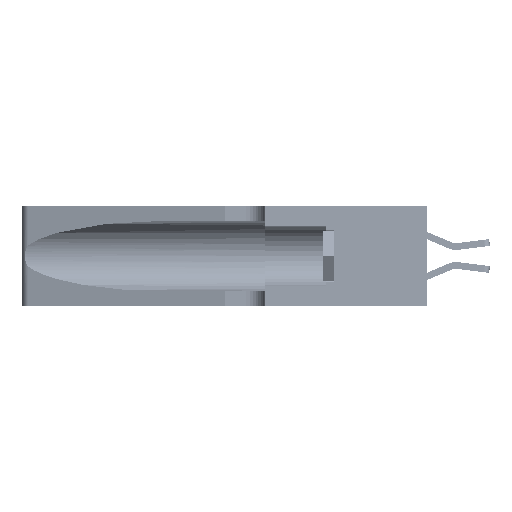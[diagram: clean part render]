
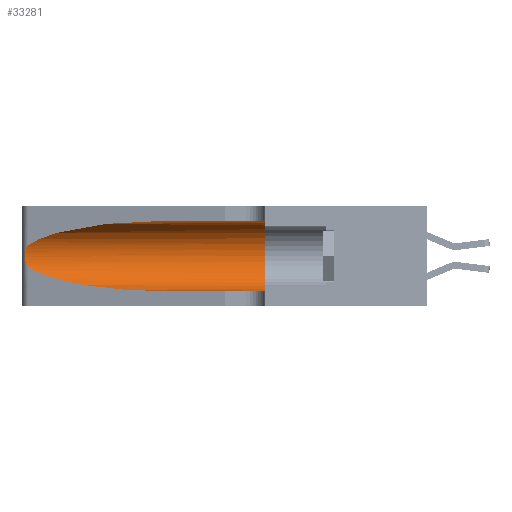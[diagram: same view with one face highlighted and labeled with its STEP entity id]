
A CAD part, left-side view. The second image highlights one B-rep face of the part: STEP entity #33281.
In plain terms, the highlighted cylindrical face has radius 3.308 mm (diameter 6.617 mm), a partial arc.
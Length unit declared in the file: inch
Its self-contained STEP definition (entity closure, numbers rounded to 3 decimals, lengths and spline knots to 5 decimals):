
#544 = VERTEX_POINT ( 'NONE', #6741 ) ;
#1522 = CARTESIAN_POINT ( 'NONE',  ( 0.25787, 1.23484, 0.2124 ) ) ;
#1813 = VERTEX_POINT ( 'NONE', #9544 ) ;
#2002 = CARTESIAN_POINT ( 'NONE',  ( 0.25487, 1.22718, 0.14631 ) ) ;
#2209 = ORIENTED_EDGE ( 'NONE', *, *, #15347, .T. ) ;
#2214 = VERTEX_POINT ( 'NONE', #2002 ) ;
#3667 = ORIENTED_EDGE ( 'NONE', *, *, #12165, .F. ) ;
#4378 = CARTESIAN_POINT ( 'NONE',  ( 0.18966, 0.96281, 0.05475 ) ) ;
#4604 = CARTESIAN_POINT ( 'NONE',  ( 0.26018, 1.23835, 0.19895 ) ) ;
#4618 = CARTESIAN_POINT ( 'NONE',  ( 0.2373, 1.15595, 0.28018 ) ) ;
#5197 = LINE ( 'NONE', #16268, #27668 ) ;
#6741 = CARTESIAN_POINT ( 'NONE',  ( 0.1305, 0.35, 0.05475 ) ) ;
#6947 = ORIENTED_EDGE ( 'NONE', *, *, #24460, .F. ) ;
#6953 = AXIS2_PLACEMENT_3D ( 'NONE', #25323, #7797, #28235 ) ;
#7427 = CARTESIAN_POINT ( 'NONE',  ( 0.1305, 0.72297, 0.05475 ) ) ;
#7623 = CARTESIAN_POINT ( 'NONE',  ( 0.26075, 1.23896, 0.178 ) ) ;
#7797 = DIRECTION ( 'NONE',  ( 0., 1., 0. ) ) ;
#9544 = CARTESIAN_POINT ( 'NONE',  ( 0.25487, 1.22718, 0.22369 ) ) ;
#10525 = DIRECTION ( 'NONE',  ( 0., -1., 0. ) ) ;
#10633 = CARTESIAN_POINT ( 'NONE',  ( 0.25856, 1.23593, 0.16098 ) ) ;
#11903 = VERTEX_POINT ( 'NONE', #29952 ) ;
#12165 = EDGE_CURVE ( 'NONE', #35425, #11903, #30650, .T. ) ;
#12490 = B_SPLINE_CURVE_WITH_KNOTS ( 'NONE', 3,
 ( #30737, #19167, #19299, #1522, #22231, #4604, #25160, #7623, #28066, #10633, #30993, #13563, #33896, #16502 ),
 .UNSPECIFIED., .F., .F.,
 ( 4, 2, 2, 2, 2, 2, 4 ),
 ( 0., 0.00027, 0.00053, 0.00107, 0.0016, 0.00187, 0.00214 ),
 .UNSPECIFIED. ) ;
#13414 = ORIENTED_EDGE ( 'NONE', *, *, #25093, .T. ) ;
#13563 = CARTESIAN_POINT ( 'NONE',  ( 0.25639, 1.23186, 0.15144 ) ) ;
#14425 = DIRECTION ( 'NONE',  ( 0., 0., -1. ) ) ;
#15304 =( BOUNDED_CURVE ( )  B_SPLINE_CURVE ( 3, ( #19084, #22009, #4378, #24947 ),
 .UNSPECIFIED., .F., .T. ) 
 B_SPLINE_CURVE_WITH_KNOTS ( ( 4, 4 ),
 ( 3.44316, 4.71239 ),
 .UNSPECIFIED. ) 
 CURVE ( )  GEOMETRIC_REPRESENTATION_ITEM ( )  RATIONAL_B_SPLINE_CURVE ( ( 1., 0.87, 0.87, 1. ) ) 
 REPRESENTATION_ITEM ( '' )  );
#15347 = EDGE_CURVE ( 'NONE', #35643, #544, #5197, .T. ) ;
#15364 = EDGE_CURVE ( 'NONE', #35425, #1813, #35540, .T. ) ;
#16268 = CARTESIAN_POINT ( 'NONE',  ( 0.1305, 1.61858, 0.05475 ) ) ;
#16392 = CARTESIAN_POINT ( 'NONE',  ( 0.18966, 0.96281, 0.31525 ) ) ;
#16502 = CARTESIAN_POINT ( 'NONE',  ( 0.25487, 1.22718, 0.14631 ) ) ;
#17338 = CARTESIAN_POINT ( 'NONE',  ( 0.1305, 1.61858, 0.185 ) ) ;
#18422 = ORIENTED_EDGE ( 'NONE', *, *, #15364, .T. ) ;
#19084 = CARTESIAN_POINT ( 'NONE',  ( 0.25487, 1.22718, 0.14631 ) ) ;
#19167 = CARTESIAN_POINT ( 'NONE',  ( 0.25555, 1.22994, 0.2215 ) ) ;
#19299 = CARTESIAN_POINT ( 'NONE',  ( 0.25639, 1.23184, 0.21858 ) ) ;
#19638 = DIRECTION ( 'NONE',  ( 0., -1., 0. ) ) ;
#19976 = EDGE_CURVE ( 'NONE', #2214, #35643, #15304, .T. ) ;
#20464 = CIRCLE ( 'NONE', #6953, 0.13025 ) ;
#22009 = CARTESIAN_POINT ( 'NONE',  ( 0.2373, 1.15595, 0.08982 ) ) ;
#22231 = CARTESIAN_POINT ( 'NONE',  ( 0.25854, 1.2359, 0.20912 ) ) ;
#24092 = AXIS2_PLACEMENT_3D ( 'NONE', #17338, #28919, #14425 ) ;
#24460 = EDGE_CURVE ( 'NONE', #11903, #544, #20464, .T. ) ;
#24822 = ORIENTED_EDGE ( 'NONE', *, *, #19976, .T. ) ;
#24947 = CARTESIAN_POINT ( 'NONE',  ( 0.1305, 0.72297, 0.05475 ) ) ;
#25093 = EDGE_CURVE ( 'NONE', #1813, #2214, #12490, .T. ) ;
#25160 = CARTESIAN_POINT ( 'NONE',  ( 0.26075, 1.23896, 0.19203 ) ) ;
#25179 = CARTESIAN_POINT ( 'NONE',  ( 0.25487, 1.22718, 0.22369 ) ) ;
#25323 = CARTESIAN_POINT ( 'NONE',  ( 0.1305, 0.35, 0.185 ) ) ;
#27668 = VECTOR ( 'NONE', #10525, 39.37008 ) ;
#28066 = CARTESIAN_POINT ( 'NONE',  ( 0.26017, 1.23833, 0.17102 ) ) ;
#28235 = DIRECTION ( 'NONE',  ( 0., 0., 1. ) ) ;
#28281 = EDGE_LOOP ( 'NONE', ( #18422, #13414, #24822, #2209, #6947, #3667 ) ) ;
#28919 = DIRECTION ( 'NONE',  ( 0., -1., 0. ) ) ;
#29952 = CARTESIAN_POINT ( 'NONE',  ( 0.1305, 0.35, 0.31525 ) ) ;
#29991 = FACE_OUTER_BOUND ( 'NONE', #28281, .T. ) ;
#30650 = LINE ( 'NONE', #37005, #37443 ) ;
#30737 = CARTESIAN_POINT ( 'NONE',  ( 0.25487, 1.22718, 0.22369 ) ) ;
#30993 = CARTESIAN_POINT ( 'NONE',  ( 0.25789, 1.23486, 0.15765 ) ) ;
#32589 = CARTESIAN_POINT ( 'NONE',  ( 0.1305, 0.72297, 0.31525 ) ) ;
#33281 = ADVANCED_FACE ( 'NONE', ( #29991 ), #36776, .F. ) ;
#33773 = CARTESIAN_POINT ( 'NONE',  ( 0.1305, 0.72297, 0.31525 ) ) ;
#33896 = CARTESIAN_POINT ( 'NONE',  ( 0.25555, 1.22993, 0.14849 ) ) ;
#35425 = VERTEX_POINT ( 'NONE', #32589 ) ;
#35540 =( BOUNDED_CURVE ( )  B_SPLINE_CURVE ( 3, ( #33773, #16392, #4618, #25179 ),
 .UNSPECIFIED., .F., .F. ) 
 B_SPLINE_CURVE_WITH_KNOTS ( ( 4, 4 ),
 ( 1.5708, 2.84003 ),
 .UNSPECIFIED. ) 
 CURVE ( )  GEOMETRIC_REPRESENTATION_ITEM ( )  RATIONAL_B_SPLINE_CURVE ( ( 1., 0.87, 0.87, 1. ) ) 
 REPRESENTATION_ITEM ( '' )  );
#35643 = VERTEX_POINT ( 'NONE', #7427 ) ;
#36776 = CYLINDRICAL_SURFACE ( 'NONE', #24092, 0.13025 ) ;
#37005 = CARTESIAN_POINT ( 'NONE',  ( 0.1305, 1.61858, 0.31525 ) ) ;
#37443 = VECTOR ( 'NONE', #19638, 39.37008 ) ;
